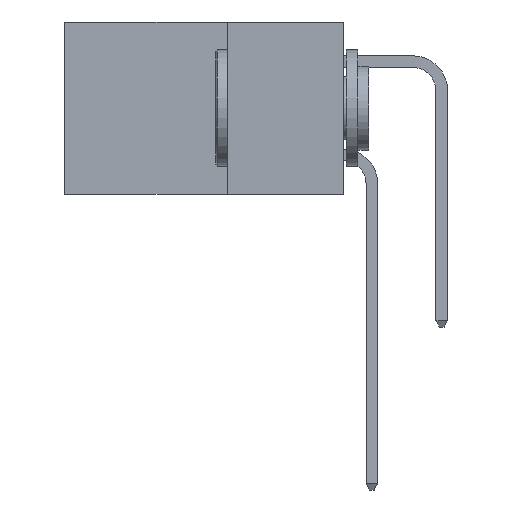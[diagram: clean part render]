
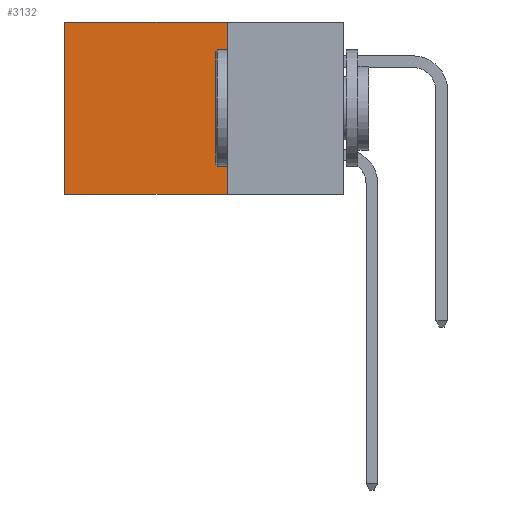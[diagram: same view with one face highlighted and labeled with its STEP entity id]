
A CAD part, left-side view. The second image highlights one B-rep face of the part: STEP entity #3132.
In plain terms, the highlighted planar face has unit normal (-1, 0, 0).
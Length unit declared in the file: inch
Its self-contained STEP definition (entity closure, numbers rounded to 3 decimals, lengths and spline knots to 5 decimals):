
#212 = CARTESIAN_POINT ( 'NONE',  ( 0.2615, 0.25, 0. ) ) ;
#541 = CARTESIAN_POINT ( 'NONE',  ( 0.2615, 0.6, -0.37 ) ) ;
#916 = VECTOR ( 'NONE', #13143, 39.37008 ) ;
#2226 = CARTESIAN_POINT ( 'NONE',  ( 0.2615, 0.25, 0. ) ) ;
#2870 = FACE_OUTER_BOUND ( 'NONE', #2938, .T. ) ;
#2938 = EDGE_LOOP ( 'NONE', ( #7822, #11971, #9491, #8249 ) ) ;
#3066 = CARTESIAN_POINT ( 'NONE',  ( 0.2615, 0.6, 0. ) ) ;
#3132 = ADVANCED_FACE ( 'NONE', ( #2870 ), #9357, .F. ) ;
#4548 = LINE ( 'NONE', #212, #12587 ) ;
#6294 = VECTOR ( 'NONE', #8980, 39.37008 ) ;
#6630 = LINE ( 'NONE', #7875, #6294 ) ;
#7071 = EDGE_CURVE ( 'NONE', #8289, #9100, #9500, .T. ) ;
#7140 = AXIS2_PLACEMENT_3D ( 'NONE', #9305, #9042, #8978 ) ;
#7241 = VERTEX_POINT ( 'NONE', #541 ) ;
#7660 = DIRECTION ( 'NONE',  ( 0., 1., 0. ) ) ;
#7822 = ORIENTED_EDGE ( 'NONE', *, *, #8324, .T. ) ;
#7875 = CARTESIAN_POINT ( 'NONE',  ( 0.2615, 0.6, -0.37 ) ) ;
#8249 = ORIENTED_EDGE ( 'NONE', *, *, #13317, .T. ) ;
#8289 = VERTEX_POINT ( 'NONE', #2226 ) ;
#8324 = EDGE_CURVE ( 'NONE', #9279, #7241, #6630, .T. ) ;
#8779 = CARTESIAN_POINT ( 'NONE',  ( 0.2615, 0.25, -0.37 ) ) ;
#8978 = DIRECTION ( 'NONE',  ( 0., 0., -1. ) ) ;
#8980 = DIRECTION ( 'NONE',  ( 0., 0., -1. ) ) ;
#9042 = DIRECTION ( 'NONE',  ( 1., 0., 0. ) ) ;
#9100 = VERTEX_POINT ( 'NONE', #11295 ) ;
#9279 = VERTEX_POINT ( 'NONE', #3066 ) ;
#9305 = CARTESIAN_POINT ( 'NONE',  ( 0.2615, 0.25, -0.37 ) ) ;
#9357 = PLANE ( 'NONE',  #7140 ) ;
#9491 = ORIENTED_EDGE ( 'NONE', *, *, #7071, .F. ) ;
#9500 = LINE ( 'NONE', #8779, #11908 ) ;
#9792 = LINE ( 'NONE', #12174, #916 ) ;
#9874 = DIRECTION ( 'NONE',  ( 0., 0., -1. ) ) ;
#11126 = EDGE_CURVE ( 'NONE', #9100, #7241, #9792, .T. ) ;
#11295 = CARTESIAN_POINT ( 'NONE',  ( 0.2615, 0.25, -0.37 ) ) ;
#11908 = VECTOR ( 'NONE', #9874, 39.37008 ) ;
#11971 = ORIENTED_EDGE ( 'NONE', *, *, #11126, .F. ) ;
#12174 = CARTESIAN_POINT ( 'NONE',  ( 0.2615, 0.25, -0.37 ) ) ;
#12587 = VECTOR ( 'NONE', #7660, 39.37008 ) ;
#13143 = DIRECTION ( 'NONE',  ( 0., 1., 0. ) ) ;
#13317 = EDGE_CURVE ( 'NONE', #8289, #9279, #4548, .T. ) ;
